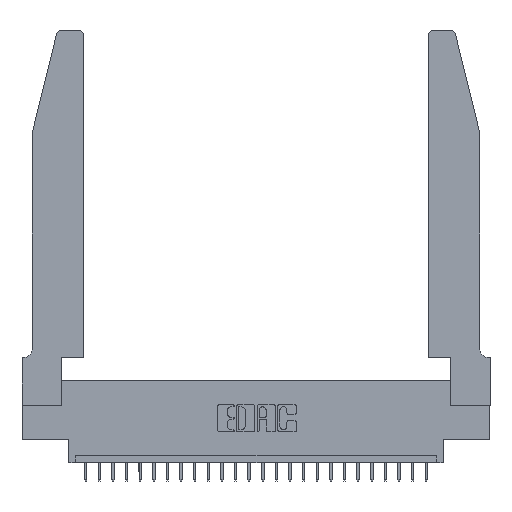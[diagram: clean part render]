
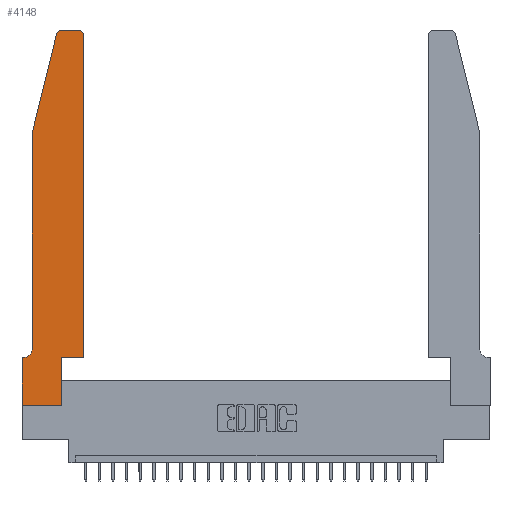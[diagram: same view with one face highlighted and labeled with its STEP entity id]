
A CAD part, top view. The second image highlights one B-rep face of the part: STEP entity #4148.
In plain terms, the highlighted planar face has unit normal (0, 0, 1).
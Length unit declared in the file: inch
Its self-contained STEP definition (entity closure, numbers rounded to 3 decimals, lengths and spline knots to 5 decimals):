
#286 = VECTOR ( 'NONE', #16079, 39.37008 ) ;
#428 = CARTESIAN_POINT ( 'NONE',  ( 0., 0., 0.37 ) ) ;
#535 = LINE ( 'NONE', #4995, #5306 ) ;
#856 = ORIENTED_EDGE ( 'NONE', *, *, #8740, .T. ) ;
#1159 = DIRECTION ( 'NONE',  ( -0.239, -0.971, 0. ) ) ;
#1287 = CARTESIAN_POINT ( 'NONE',  ( 0.4505, 0.35, 0.37 ) ) ;
#1743 = DIRECTION ( 'NONE',  ( 0., 0., -1. ) ) ;
#1928 = DIRECTION ( 'NONE',  ( 0., 0., 1. ) ) ;
#2381 = ORIENTED_EDGE ( 'NONE', *, *, #23629, .T. ) ;
#3119 = VERTEX_POINT ( 'NONE', #15531 ) ;
#3127 = LINE ( 'NONE', #3653, #3263 ) ;
#3263 = VECTOR ( 'NONE', #17827, 39.37008 ) ;
#3400 = CARTESIAN_POINT ( 'NONE',  ( 0.2865, 0.35, 0.37 ) ) ;
#3653 = CARTESIAN_POINT ( 'NONE',  ( 0.4505, 0.35, 0.37 ) ) ;
#3699 = CARTESIAN_POINT ( 'NONE',  ( 0.284, 2.72, 0.37 ) ) ;
#4028 = EDGE_CURVE ( 'NONE', #5825, #3119, #20601, .T. ) ;
#4148 = ADVANCED_FACE ( 'NONE', ( #10558 ), #24753, .T. ) ;
#4806 = LINE ( 'NONE', #23589, #14863 ) ;
#4995 = CARTESIAN_POINT ( 'NONE',  ( 0.0755, 0.35, 0.37 ) ) ;
#5306 = VECTOR ( 'NONE', #13081, 39.37008 ) ;
#5598 = DIRECTION ( 'NONE',  ( 1., 0., 0. ) ) ;
#5825 = VERTEX_POINT ( 'NONE', #19041 ) ;
#5888 = ORIENTED_EDGE ( 'NONE', *, *, #11820, .T. ) ;
#5894 = CIRCLE ( 'NONE', #18837, 0.03 ) ;
#6462 = DIRECTION ( 'NONE',  ( 1., 0., 0. ) ) ;
#7708 = LINE ( 'NONE', #3400, #286 ) ;
#7942 = DIRECTION ( 'NONE',  ( -1., 0., 0. ) ) ;
#8578 = CARTESIAN_POINT ( 'NONE',  ( 0.0755, 0.42, 0.37 ) ) ;
#8740 = EDGE_CURVE ( 'NONE', #20185, #9517, #20238, .T. ) ;
#8826 = VECTOR ( 'NONE', #18596, 39.37008 ) ;
#9031 = DIRECTION ( 'NONE',  ( 0., -1., 0. ) ) ;
#9428 = ORIENTED_EDGE ( 'NONE', *, *, #12829, .T. ) ;
#9517 = VERTEX_POINT ( 'NONE', #19040 ) ;
#9534 = EDGE_CURVE ( 'NONE', #14072, #19141, #535, .T. ) ;
#9716 = DIRECTION ( 'NONE',  ( -1., 0., 0. ) ) ;
#10079 = VECTOR ( 'NONE', #6462, 39.37008 ) ;
#10164 = CIRCLE ( 'NONE', #14929, 0.07 ) ;
#10352 = CARTESIAN_POINT ( 'NONE',  ( 0., 0., 0.37 ) ) ;
#10558 = FACE_OUTER_BOUND ( 'NONE', #17726, .T. ) ;
#10606 = VERTEX_POINT ( 'NONE', #1287 ) ;
#10655 = CARTESIAN_POINT ( 'NONE',  ( 0.0755, 2., 0.37 ) ) ;
#11163 = CARTESIAN_POINT ( 'NONE',  ( 0.25487, 2.72718, 0.37 ) ) ;
#11168 = VERTEX_POINT ( 'NONE', #13794 ) ;
#11715 = ORIENTED_EDGE ( 'NONE', *, *, #26699, .T. ) ;
#11820 = EDGE_CURVE ( 'NONE', #18248, #13796, #4806, .T. ) ;
#11919 = DIRECTION ( 'NONE',  ( 0., 0., 1. ) ) ;
#12115 = CARTESIAN_POINT ( 'NONE',  ( 0., 0., 0.37 ) ) ;
#12130 = CARTESIAN_POINT ( 'NONE',  ( 0.0055, 0.42, 0.37 ) ) ;
#12454 = CARTESIAN_POINT ( 'NONE',  ( 0., 0.35, 0.37 ) ) ;
#12742 = EDGE_CURVE ( 'NONE', #3119, #20661, #25928, .T. ) ;
#12829 = EDGE_CURVE ( 'NONE', #11168, #10606, #3127, .T. ) ;
#13081 = DIRECTION ( 'NONE',  ( -1., 0., 0. ) ) ;
#13794 = CARTESIAN_POINT ( 'NONE',  ( 0.2865, 0.35, 0.37 ) ) ;
#13796 = VERTEX_POINT ( 'NONE', #23824 ) ;
#13896 = CARTESIAN_POINT ( 'NONE',  ( 0.2605, 2.75, 0.37 ) ) ;
#14072 = VERTEX_POINT ( 'NONE', #26449 ) ;
#14079 = ORIENTED_EDGE ( 'NONE', *, *, #15843, .T. ) ;
#14324 = EDGE_CURVE ( 'NONE', #13796, #16788, #25246, .T. ) ;
#14403 = CARTESIAN_POINT ( 'NONE',  ( 0.4505, 0.35, 0.37 ) ) ;
#14699 = ORIENTED_EDGE ( 'NONE', *, *, #16143, .T. ) ;
#14863 = VECTOR ( 'NONE', #1159, 39.37008 ) ;
#14929 = AXIS2_PLACEMENT_3D ( 'NONE', #12130, #1743, #7942 ) ;
#15531 = CARTESIAN_POINT ( 'NONE',  ( 0.4205, 2.75, 0.37 ) ) ;
#15843 = EDGE_CURVE ( 'NONE', #20661, #18248, #5894, .T. ) ;
#16079 = DIRECTION ( 'NONE',  ( 0., 1., 0. ) ) ;
#16143 = EDGE_CURVE ( 'NONE', #9517, #11168, #7708, .T. ) ;
#16770 = ORIENTED_EDGE ( 'NONE', *, *, #9534, .T. ) ;
#16788 = VERTEX_POINT ( 'NONE', #8578 ) ;
#16878 = ORIENTED_EDGE ( 'NONE', *, *, #14324, .T. ) ;
#17726 = EDGE_LOOP ( 'NONE', ( #18308, #14079, #5888, #16878, #11715, #16770, #25371, #856, #14699, #9428, #2381, #25046 ) ) ;
#17827 = DIRECTION ( 'NONE',  ( 1., 0., 0. ) ) ;
#17870 = DIRECTION ( 'NONE',  ( 0., 0., 1. ) ) ;
#18248 = VERTEX_POINT ( 'NONE', #11163 ) ;
#18308 = ORIENTED_EDGE ( 'NONE', *, *, #12742, .T. ) ;
#18540 = DIRECTION ( 'NONE',  ( 1., 0., 0. ) ) ;
#18596 = DIRECTION ( 'NONE',  ( 0., -1., 0. ) ) ;
#18837 = AXIS2_PLACEMENT_3D ( 'NONE', #3699, #11919, #20178 ) ;
#18859 = VECTOR ( 'NONE', #9031, 39.37008 ) ;
#19040 = CARTESIAN_POINT ( 'NONE',  ( 0.2865, 0., 0.37 ) ) ;
#19041 = CARTESIAN_POINT ( 'NONE',  ( 0.4505, 2.72, 0.37 ) ) ;
#19141 = VERTEX_POINT ( 'NONE', #24053 ) ;
#19725 = AXIS2_PLACEMENT_3D ( 'NONE', #19771, #17870, #5598 ) ;
#19771 = CARTESIAN_POINT ( 'NONE',  ( 0.4205, 2.72, 0.37 ) ) ;
#20178 = DIRECTION ( 'NONE',  ( 1., 0., 0. ) ) ;
#20185 = VERTEX_POINT ( 'NONE', #428 ) ;
#20238 = LINE ( 'NONE', #12115, #10079 ) ;
#20601 = CIRCLE ( 'NONE', #19725, 0.03 ) ;
#20661 = VERTEX_POINT ( 'NONE', #23755 ) ;
#23100 = VECTOR ( 'NONE', #9716, 39.37008 ) ;
#23589 = CARTESIAN_POINT ( 'NONE',  ( 0.0755, 2., 0.37 ) ) ;
#23629 = EDGE_CURVE ( 'NONE', #10606, #5825, #26703, .T. ) ;
#23755 = CARTESIAN_POINT ( 'NONE',  ( 0.284, 2.75, 0.37 ) ) ;
#23824 = CARTESIAN_POINT ( 'NONE',  ( 0.0755, 2., 0.37 ) ) ;
#24053 = CARTESIAN_POINT ( 'NONE',  ( 0., 0.35, 0.37 ) ) ;
#24157 = LINE ( 'NONE', #10352, #8826 ) ;
#24753 = PLANE ( 'NONE',  #26625 ) ;
#24809 = DIRECTION ( 'NONE',  ( 0., 1., 0. ) ) ;
#24926 = EDGE_CURVE ( 'NONE', #19141, #20185, #24157, .T. ) ;
#25046 = ORIENTED_EDGE ( 'NONE', *, *, #4028, .T. ) ;
#25246 = LINE ( 'NONE', #10655, #18859 ) ;
#25371 = ORIENTED_EDGE ( 'NONE', *, *, #24926, .T. ) ;
#25928 = LINE ( 'NONE', #13896, #23100 ) ;
#26010 = VECTOR ( 'NONE', #24809, 39.37008 ) ;
#26449 = CARTESIAN_POINT ( 'NONE',  ( 0.0055, 0.35, 0.37 ) ) ;
#26625 = AXIS2_PLACEMENT_3D ( 'NONE', #12454, #1928, #18540 ) ;
#26699 = EDGE_CURVE ( 'NONE', #16788, #14072, #10164, .T. ) ;
#26703 = LINE ( 'NONE', #14403, #26010 ) ;
